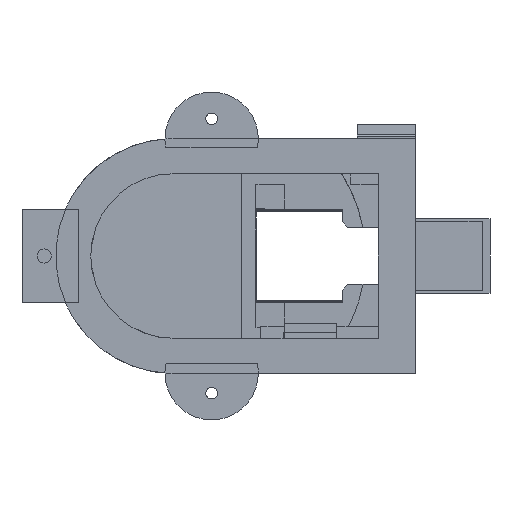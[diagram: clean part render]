
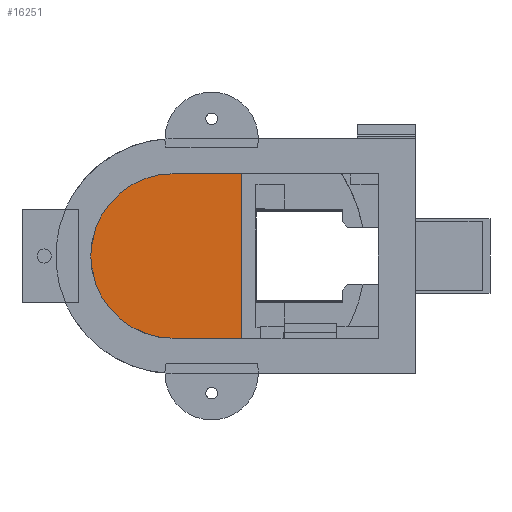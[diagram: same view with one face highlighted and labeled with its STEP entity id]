
A CAD part, left-side view. The second image highlights one B-rep face of the part: STEP entity #16251.
In plain terms, the highlighted planar face has unit normal (-1, 0, 0).
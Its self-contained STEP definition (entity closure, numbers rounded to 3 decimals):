
#1947 = PLANE('',#1948);
#1948 = AXIS2_PLACEMENT_3D('',#1949,#1950,#1951);
#1949 = CARTESIAN_POINT('',(-19.05,47.913,14.1));
#1950 = DIRECTION('',(0.,0.,1.));
#1951 = DIRECTION('',(0.,-1.,0.));
#2688 = CYLINDRICAL_SURFACE('',#2689,14.1);
#2689 = AXIS2_PLACEMENT_3D('',#2690,#2691,#2692);
#2690 = CARTESIAN_POINT('',(-19.05,47.913,0.));
#2691 = DIRECTION('',(1.,0.,0.));
#2692 = DIRECTION('',(0.,-1.,0.));
#2859 = PLANE('',#2860);
#2860 = AXIS2_PLACEMENT_3D('',#2861,#2862,#2863);
#2861 = CARTESIAN_POINT('',(-19.05,6.363,-14.1));
#2862 = DIRECTION('',(0.,0.,-1.));
#2863 = DIRECTION('',(0.,1.,0.));
#6853 = EDGE_CURVE('',#6854,#6856,#6858,.T.);
#6854 = VERTEX_POINT('',#6855);
#6855 = CARTESIAN_POINT('',(-19.05,47.913,14.1));
#6856 = VERTEX_POINT('',#6857);
#6857 = CARTESIAN_POINT('',(-19.05,36.099,14.1));
#6858 = SURFACE_CURVE('',#6859,(#6863,#6870),.PCURVE_S1.);
#6859 = LINE('',#6860,#6861);
#6860 = CARTESIAN_POINT('',(-19.05,47.913,14.1));
#6861 = VECTOR('',#6862,1.);
#6862 = DIRECTION('',(0.,-1.,0.));
#6863 = PCURVE('',#1947,#6864);
#6864 = DEFINITIONAL_REPRESENTATION('',(#6865),#6869);
#6865 = LINE('',#6866,#6867);
#6866 = CARTESIAN_POINT('',(0.,0.));
#6867 = VECTOR('',#6868,1.);
#6868 = DIRECTION('',(1.,0.));
#6869 = ( GEOMETRIC_REPRESENTATION_CONTEXT(2) 
PARAMETRIC_REPRESENTATION_CONTEXT() REPRESENTATION_CONTEXT('2D SPACE',''
  ) );
#6870 = PCURVE('',#6871,#6876);
#6871 = PLANE('',#6872);
#6872 = AXIS2_PLACEMENT_3D('',#6873,#6874,#6875);
#6873 = CARTESIAN_POINT('',(-19.05,13.081,-15.431));
#6874 = DIRECTION('',(-1.,0.,0.));
#6875 = DIRECTION('',(0.,0.,-1.));
#6876 = DEFINITIONAL_REPRESENTATION('',(#6877),#6881);
#6877 = LINE('',#6878,#6879);
#6878 = CARTESIAN_POINT('',(-29.531,-34.832));
#6879 = VECTOR('',#6880,1.);
#6880 = DIRECTION('',(0.,1.));
#6881 = ( GEOMETRIC_REPRESENTATION_CONTEXT(2) 
PARAMETRIC_REPRESENTATION_CONTEXT() REPRESENTATION_CONTEXT('2D SPACE',''
  ) );
#8278 = EDGE_CURVE('',#6854,#8279,#8281,.T.);
#8279 = VERTEX_POINT('',#8280);
#8280 = CARTESIAN_POINT('',(-19.05,47.913,-14.1));
#8281 = SURFACE_CURVE('',#8282,(#8287,#8294),.PCURVE_S1.);
#8282 = CIRCLE('',#8283,14.1);
#8283 = AXIS2_PLACEMENT_3D('',#8284,#8285,#8286);
#8284 = CARTESIAN_POINT('',(-19.05,47.913,0.));
#8285 = DIRECTION('',(-1.,0.,0.));
#8286 = DIRECTION('',(0.,-1.,0.));
#8287 = PCURVE('',#2688,#8288);
#8288 = DEFINITIONAL_REPRESENTATION('',(#8289),#8293);
#8289 = LINE('',#8290,#8291);
#8290 = CARTESIAN_POINT('',(6.283,0.));
#8291 = VECTOR('',#8292,1.);
#8292 = DIRECTION('',(-1.,0.));
#8293 = ( GEOMETRIC_REPRESENTATION_CONTEXT(2) 
PARAMETRIC_REPRESENTATION_CONTEXT() REPRESENTATION_CONTEXT('2D SPACE',''
  ) );
#8294 = PCURVE('',#6871,#8295);
#8295 = DEFINITIONAL_REPRESENTATION('',(#8296),#8300);
#8296 = CIRCLE('',#8297,14.1);
#8297 = AXIS2_PLACEMENT_2D('',#8298,#8299);
#8298 = CARTESIAN_POINT('',(-15.431,-34.832));
#8299 = DIRECTION('',(0.,1.));
#8300 = ( GEOMETRIC_REPRESENTATION_CONTEXT(2) 
PARAMETRIC_REPRESENTATION_CONTEXT() REPRESENTATION_CONTEXT('2D SPACE',''
  ) );
#11013 = EDGE_CURVE('',#11014,#8279,#11016,.T.);
#11014 = VERTEX_POINT('',#11015);
#11015 = CARTESIAN_POINT('',(-19.05,36.099,-14.1));
#11016 = SURFACE_CURVE('',#11017,(#11021,#11028),.PCURVE_S1.);
#11017 = LINE('',#11018,#11019);
#11018 = CARTESIAN_POINT('',(-19.05,6.363,-14.1));
#11019 = VECTOR('',#11020,1.);
#11020 = DIRECTION('',(0.,1.,0.));
#11021 = PCURVE('',#2859,#11022);
#11022 = DEFINITIONAL_REPRESENTATION('',(#11023),#11027);
#11023 = LINE('',#11024,#11025);
#11024 = CARTESIAN_POINT('',(0.,0.));
#11025 = VECTOR('',#11026,1.);
#11026 = DIRECTION('',(1.,0.));
#11027 = ( GEOMETRIC_REPRESENTATION_CONTEXT(2) 
PARAMETRIC_REPRESENTATION_CONTEXT() REPRESENTATION_CONTEXT('2D SPACE',''
  ) );
#11028 = PCURVE('',#6871,#11029);
#11029 = DEFINITIONAL_REPRESENTATION('',(#11030),#11034);
#11030 = LINE('',#11031,#11032);
#11031 = CARTESIAN_POINT('',(-1.331,6.718));
#11032 = VECTOR('',#11033,1.);
#11033 = DIRECTION('',(0.,-1.));
#11034 = ( GEOMETRIC_REPRESENTATION_CONTEXT(2) 
PARAMETRIC_REPRESENTATION_CONTEXT() REPRESENTATION_CONTEXT('2D SPACE',''
  ) );
#16251 = ADVANCED_FACE('',(#16252),#6871,.T.);
#16252 = FACE_BOUND('',#16253,.T.);
#16253 = EDGE_LOOP('',(#16254,#16255,#16281,#16282));
#16254 = ORIENTED_EDGE('',*,*,#11013,.F.);
#16255 = ORIENTED_EDGE('',*,*,#16256,.F.);
#16256 = EDGE_CURVE('',#6856,#11014,#16257,.T.);
#16257 = SURFACE_CURVE('',#16258,(#16262,#16269),.PCURVE_S1.);
#16258 = LINE('',#16259,#16260);
#16259 = CARTESIAN_POINT('',(-19.05,36.099,14.667));
#16260 = VECTOR('',#16261,1.);
#16261 = DIRECTION('',(0.,0.,-1.));
#16262 = PCURVE('',#6871,#16263);
#16263 = DEFINITIONAL_REPRESENTATION('',(#16264),#16268);
#16264 = LINE('',#16265,#16266);
#16265 = CARTESIAN_POINT('',(-30.098,-23.018));
#16266 = VECTOR('',#16267,1.);
#16267 = DIRECTION('',(1.,0.));
#16268 = ( GEOMETRIC_REPRESENTATION_CONTEXT(2) 
PARAMETRIC_REPRESENTATION_CONTEXT() REPRESENTATION_CONTEXT('2D SPACE',''
  ) );
#16269 = PCURVE('',#16270,#16275);
#16270 = PLANE('',#16271);
#16271 = AXIS2_PLACEMENT_3D('',#16272,#16273,#16274);
#16272 = CARTESIAN_POINT('',(-19.05,36.099,14.667));
#16273 = DIRECTION('',(0.,1.,0.));
#16274 = DIRECTION('',(0.,0.,-1.));
#16275 = DEFINITIONAL_REPRESENTATION('',(#16276),#16280);
#16276 = LINE('',#16277,#16278);
#16277 = CARTESIAN_POINT('',(0.,0.));
#16278 = VECTOR('',#16279,1.);
#16279 = DIRECTION('',(1.,0.));
#16280 = ( GEOMETRIC_REPRESENTATION_CONTEXT(2) 
PARAMETRIC_REPRESENTATION_CONTEXT() REPRESENTATION_CONTEXT('2D SPACE',''
  ) );
#16281 = ORIENTED_EDGE('',*,*,#6853,.F.);
#16282 = ORIENTED_EDGE('',*,*,#8278,.T.);
